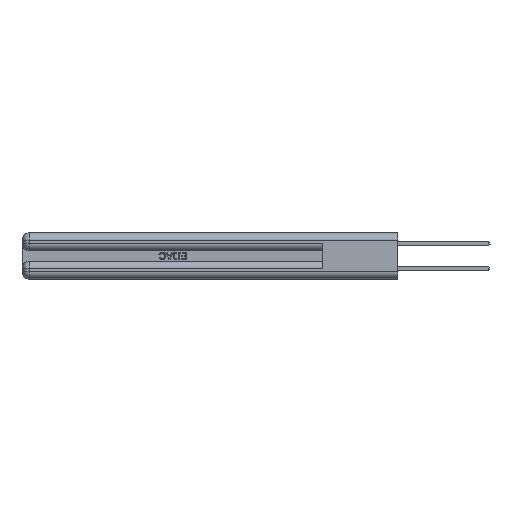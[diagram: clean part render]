
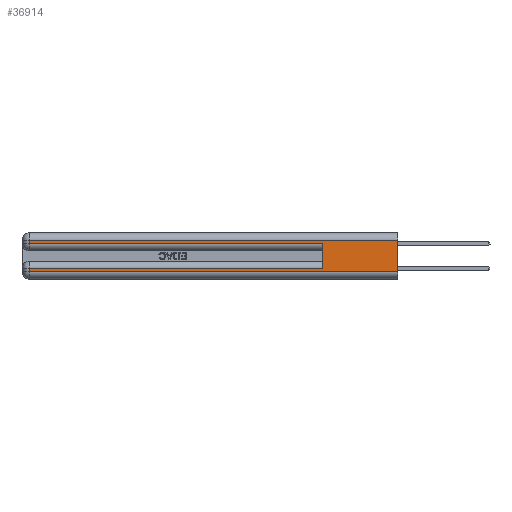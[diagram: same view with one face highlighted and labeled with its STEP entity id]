
A CAD part, left-side view. The second image highlights one B-rep face of the part: STEP entity #36914.
In plain terms, the highlighted planar face has unit normal (-1, 0, 0).
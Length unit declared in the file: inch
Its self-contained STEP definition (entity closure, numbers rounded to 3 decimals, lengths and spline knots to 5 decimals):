
#346 = CARTESIAN_POINT ( 'NONE',  ( 0., 0., 0.285 ) ) ;
#402 = CARTESIAN_POINT ( 'NONE',  ( 0., 0., 0.06 ) ) ;
#2598 = EDGE_CURVE ( 'NONE', #27036, #39799, #26953, .T. ) ;
#3007 = DIRECTION ( 'NONE',  ( 0., 0., -1. ) ) ;
#4115 = VERTEX_POINT ( 'NONE', #42060 ) ;
#4236 = EDGE_CURVE ( 'NONE', #20873, #27036, #28072, .T. ) ;
#4617 = VERTEX_POINT ( 'NONE', #9472 ) ;
#4991 = FACE_OUTER_BOUND ( 'NONE', #28574, .T. ) ;
#6056 = VERTEX_POINT ( 'NONE', #10039 ) ;
#6312 = DIRECTION ( 'NONE',  ( 0., 1., 0. ) ) ;
#6739 = PLANE ( 'NONE',  #40574 ) ;
#7046 = CARTESIAN_POINT ( 'NONE',  ( 0., 0.6, 0.085 ) ) ;
#7054 = VECTOR ( 'NONE', #27213, 39.37008 ) ;
#7079 = VECTOR ( 'NONE', #40538, 39.37008 ) ;
#7682 = VECTOR ( 'NONE', #15180, 39.37008 ) ;
#8540 = CARTESIAN_POINT ( 'NONE',  ( 0., 0., 0.31 ) ) ;
#9472 = CARTESIAN_POINT ( 'NONE',  ( 0., 2.94, 0.06 ) ) ;
#9503 = LINE ( 'NONE', #36673, #7079 ) ;
#9550 = EDGE_CURVE ( 'NONE', #42887, #45930, #37015, .T. ) ;
#10039 = CARTESIAN_POINT ( 'NONE',  ( 0., 0., 0.06 ) ) ;
#12486 = ORIENTED_EDGE ( 'NONE', *, *, #17401, .T. ) ;
#13900 = DIRECTION ( 'NONE',  ( 0., 0., -1. ) ) ;
#15180 = DIRECTION ( 'NONE',  ( 0., 1., 0. ) ) ;
#15737 = DIRECTION ( 'NONE',  ( 0., 0., -1. ) ) ;
#16076 = ORIENTED_EDGE ( 'NONE', *, *, #25333, .F. ) ;
#16608 = ORIENTED_EDGE ( 'NONE', *, *, #22242, .F. ) ;
#16709 = ORIENTED_EDGE ( 'NONE', *, *, #9550, .T. ) ;
#17401 = EDGE_CURVE ( 'NONE', #39799, #4115, #36415, .T. ) ;
#20430 = LINE ( 'NONE', #402, #29466 ) ;
#20823 = ORIENTED_EDGE ( 'NONE', *, *, #2598, .T. ) ;
#20873 = VERTEX_POINT ( 'NONE', #8540 ) ;
#22242 = EDGE_CURVE ( 'NONE', #20873, #6056, #9503, .T. ) ;
#24869 = CARTESIAN_POINT ( 'NONE',  ( 0., 0.6, 0.145 ) ) ;
#25333 = EDGE_CURVE ( 'NONE', #42887, #4115, #45222, .T. ) ;
#26023 = DIRECTION ( 'NONE',  ( 1., 0., 0. ) ) ;
#26861 = VECTOR ( 'NONE', #6312, 39.37008 ) ;
#26953 = LINE ( 'NONE', #33022, #35937 ) ;
#27036 = VERTEX_POINT ( 'NONE', #45595 ) ;
#27213 = DIRECTION ( 'NONE',  ( 0., -1., 0. ) ) ;
#27422 = ORIENTED_EDGE ( 'NONE', *, *, #4236, .T. ) ;
#28072 = LINE ( 'NONE', #30425, #7682 ) ;
#28231 = CARTESIAN_POINT ( 'NONE',  ( 0., 2.94, 0.085 ) ) ;
#28574 = EDGE_LOOP ( 'NONE', ( #16608, #27422, #20823, #12486, #16076, #16709, #44197, #28684 ) ) ;
#28684 = ORIENTED_EDGE ( 'NONE', *, *, #38349, .T. ) ;
#28724 = DIRECTION ( 'NONE',  ( 0., 0., 1. ) ) ;
#29466 = VECTOR ( 'NONE', #31312, 39.37008 ) ;
#30425 = CARTESIAN_POINT ( 'NONE',  ( 0., 0., 0.31 ) ) ;
#31312 = DIRECTION ( 'NONE',  ( 0., -1., 0. ) ) ;
#31446 = LINE ( 'NONE', #34851, #40407 ) ;
#33022 = CARTESIAN_POINT ( 'NONE',  ( 0., 2.94, 0.37 ) ) ;
#34851 = CARTESIAN_POINT ( 'NONE',  ( 0., 2.94, 0.37 ) ) ;
#35937 = VECTOR ( 'NONE', #13900, 39.37008 ) ;
#36415 = LINE ( 'NONE', #346, #7054 ) ;
#36673 = CARTESIAN_POINT ( 'NONE',  ( 0., 0., 0.37 ) ) ;
#36914 = ADVANCED_FACE ( 'NONE', ( #4991 ), #6739, .F. ) ;
#37015 = LINE ( 'NONE', #40665, #26861 ) ;
#38349 = EDGE_CURVE ( 'NONE', #4617, #6056, #20430, .T. ) ;
#39185 = CARTESIAN_POINT ( 'NONE',  ( 0., 2.94, 0.285 ) ) ;
#39799 = VERTEX_POINT ( 'NONE', #39185 ) ;
#40407 = VECTOR ( 'NONE', #15737, 39.37008 ) ;
#40538 = DIRECTION ( 'NONE',  ( 0., 0., -1. ) ) ;
#40574 = AXIS2_PLACEMENT_3D ( 'NONE', #48964, #26023, #3007 ) ;
#40665 = CARTESIAN_POINT ( 'NONE',  ( 0., 0., 0.085 ) ) ;
#42060 = CARTESIAN_POINT ( 'NONE',  ( 0., 0.6, 0.285 ) ) ;
#42887 = VERTEX_POINT ( 'NONE', #7046 ) ;
#44197 = ORIENTED_EDGE ( 'NONE', *, *, #47415, .T. ) ;
#45222 = LINE ( 'NONE', #24869, #47634 ) ;
#45595 = CARTESIAN_POINT ( 'NONE',  ( 0., 2.94, 0.31 ) ) ;
#45930 = VERTEX_POINT ( 'NONE', #28231 ) ;
#47415 = EDGE_CURVE ( 'NONE', #45930, #4617, #31446, .T. ) ;
#47634 = VECTOR ( 'NONE', #28724, 39.37008 ) ;
#48964 = CARTESIAN_POINT ( 'NONE',  ( 0., 0., 0.37 ) ) ;
